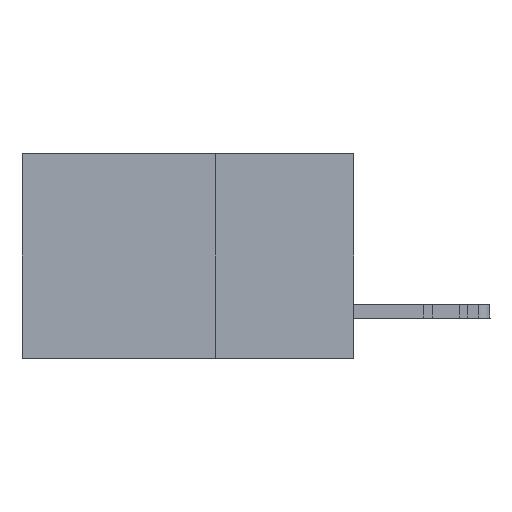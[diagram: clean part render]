
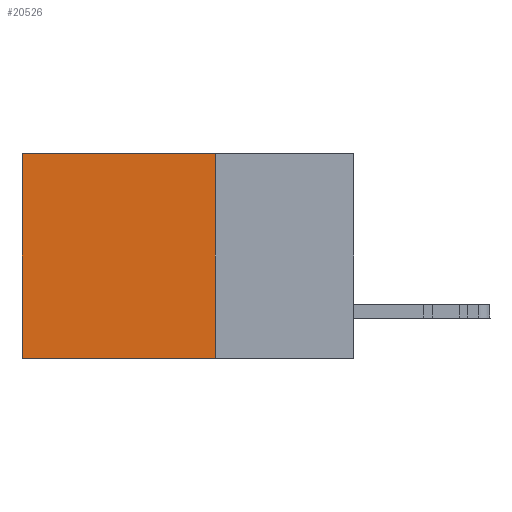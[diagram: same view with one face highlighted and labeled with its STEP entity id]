
A CAD part, left-side view. The second image highlights one B-rep face of the part: STEP entity #20526.
In plain terms, the highlighted planar face has unit normal (-1, 0, 0).
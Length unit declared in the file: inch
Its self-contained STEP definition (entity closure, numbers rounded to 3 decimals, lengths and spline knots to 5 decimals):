
#1351 = VERTEX_POINT ( 'NONE', #8201 ) ;
#1669 = CARTESIAN_POINT ( 'NONE',  ( 0.2875, 0.6, -0.37 ) ) ;
#2204 = EDGE_LOOP ( 'NONE', ( #37957, #13201, #38201, #29575 ) ) ;
#3972 = AXIS2_PLACEMENT_3D ( 'NONE', #13073, #39698, #6133 ) ;
#5847 = LINE ( 'NONE', #13239, #24204 ) ;
#6133 = DIRECTION ( 'NONE',  ( 0., 0., -1. ) ) ;
#6418 = CARTESIAN_POINT ( 'NONE',  ( 0.2875, 0.6, 0. ) ) ;
#7704 = EDGE_CURVE ( 'NONE', #1351, #15589, #34323, .T. ) ;
#8201 = CARTESIAN_POINT ( 'NONE',  ( 0.2875, 0.25, 0. ) ) ;
#9054 = PLANE ( 'NONE',  #3972 ) ;
#10385 = VECTOR ( 'NONE', #21841, 39.37008 ) ;
#11338 = EDGE_CURVE ( 'NONE', #37629, #20424, #35358, .T. ) ;
#13073 = CARTESIAN_POINT ( 'NONE',  ( 0.2875, 0.25, 0. ) ) ;
#13201 = ORIENTED_EDGE ( 'NONE', *, *, #23981, .F. ) ;
#13239 = CARTESIAN_POINT ( 'NONE',  ( 0.2875, 0.25, -0.37 ) ) ;
#13464 = EDGE_CURVE ( 'NONE', #1351, #37629, #30578, .T. ) ;
#15589 = VERTEX_POINT ( 'NONE', #23009 ) ;
#17181 = DIRECTION ( 'NONE',  ( 0., 0., -1. ) ) ;
#20044 = VECTOR ( 'NONE', #17181, 39.37008 ) ;
#20050 = FACE_OUTER_BOUND ( 'NONE', #2204, .T. ) ;
#20424 = VERTEX_POINT ( 'NONE', #1669 ) ;
#20526 = ADVANCED_FACE ( 'NONE', ( #20050 ), #9054, .F. ) ;
#21841 = DIRECTION ( 'NONE',  ( 0., 0., -1. ) ) ;
#23009 = CARTESIAN_POINT ( 'NONE',  ( 0.2875, 0.25, -0.37 ) ) ;
#23143 = DIRECTION ( 'NONE',  ( 0., 1., 0. ) ) ;
#23620 = DIRECTION ( 'NONE',  ( 0., 1., 0. ) ) ;
#23981 = EDGE_CURVE ( 'NONE', #15589, #20424, #5847, .T. ) ;
#24204 = VECTOR ( 'NONE', #23620, 39.37008 ) ;
#27417 = CARTESIAN_POINT ( 'NONE',  ( 0.2875, 0.25, 0. ) ) ;
#29575 = ORIENTED_EDGE ( 'NONE', *, *, #13464, .T. ) ;
#30578 = LINE ( 'NONE', #27417, #37665 ) ;
#34323 = LINE ( 'NONE', #37695, #20044 ) ;
#35358 = LINE ( 'NONE', #38306, #10385 ) ;
#37629 = VERTEX_POINT ( 'NONE', #6418 ) ;
#37665 = VECTOR ( 'NONE', #23143, 39.37008 ) ;
#37695 = CARTESIAN_POINT ( 'NONE',  ( 0.2875, 0.25, 0. ) ) ;
#37957 = ORIENTED_EDGE ( 'NONE', *, *, #11338, .T. ) ;
#38201 = ORIENTED_EDGE ( 'NONE', *, *, #7704, .F. ) ;
#38306 = CARTESIAN_POINT ( 'NONE',  ( 0.2875, 0.6, 0. ) ) ;
#39698 = DIRECTION ( 'NONE',  ( 1., 0., 0. ) ) ;
